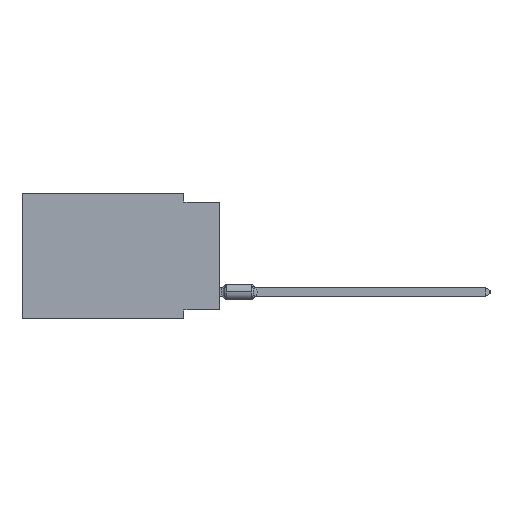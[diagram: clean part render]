
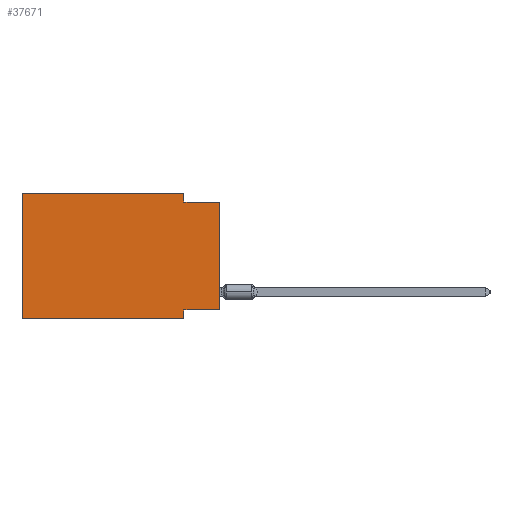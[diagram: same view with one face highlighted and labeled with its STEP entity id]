
A CAD part, left-side view. The second image highlights one B-rep face of the part: STEP entity #37671.
In plain terms, the highlighted planar face has unit normal (-1, 0, 0).
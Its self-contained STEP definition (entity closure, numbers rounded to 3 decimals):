
#9 = EDGE_CURVE ( 'NONE', #63731, #5928, #62238, .T. ) ;
#2051 = CARTESIAN_POINT ( 'NONE',  ( 0., 13.97, -8.89 ) ) ;
#3689 = VECTOR ( 'NONE', #49801, 1000. ) ;
#4534 = EDGE_CURVE ( 'NONE', #6087, #34303, #14583, .T. ) ;
#5928 = VERTEX_POINT ( 'NONE', #48019 ) ;
#6087 = VERTEX_POINT ( 'NONE', #49820 ) ;
#7218 = CARTESIAN_POINT ( 'NONE',  ( 0., 2.54, 0. ) ) ;
#8438 = VERTEX_POINT ( 'NONE', #85431 ) ;
#8828 = CARTESIAN_POINT ( 'NONE',  ( 0., 2.54, -8.89 ) ) ;
#9376 = LINE ( 'NONE', #2051, #74535 ) ;
#9816 = DIRECTION ( 'NONE',  ( 0., -1., 0. ) ) ;
#10262 = ORIENTED_EDGE ( 'NONE', *, *, #72027, .T. ) ;
#13030 = DIRECTION ( 'NONE',  ( 0., 0., -1. ) ) ;
#13647 = VECTOR ( 'NONE', #82854, 1000. ) ;
#14145 = CARTESIAN_POINT ( 'NONE',  ( 0., 0., -0.635 ) ) ;
#14396 = FACE_OUTER_BOUND ( 'NONE', #84794, .T. ) ;
#14546 = VECTOR ( 'NONE', #19195, 1000. ) ;
#14583 = LINE ( 'NONE', #14145, #59259 ) ;
#15708 = DIRECTION ( 'NONE',  ( 0., 0., -1. ) ) ;
#19195 = DIRECTION ( 'NONE',  ( 0., 1., 0. ) ) ;
#19490 = ORIENTED_EDGE ( 'NONE', *, *, #38370, .F. ) ;
#19986 = ORIENTED_EDGE ( 'NONE', *, *, #29115, .F. ) ;
#23646 = CARTESIAN_POINT ( 'NONE',  ( 0., 2.54, -8.89 ) ) ;
#23866 = CARTESIAN_POINT ( 'NONE',  ( 0., 0., -0.635 ) ) ;
#24412 = ORIENTED_EDGE ( 'NONE', *, *, #4534, .F. ) ;
#24677 = VERTEX_POINT ( 'NONE', #23646 ) ;
#25550 = EDGE_CURVE ( 'NONE', #63731, #34303, #51093, .T. ) ;
#27673 = PLANE ( 'NONE',  #41561 ) ;
#29115 = EDGE_CURVE ( 'NONE', #5928, #24677, #35381, .T. ) ;
#34303 = VERTEX_POINT ( 'NONE', #23866 ) ;
#34336 = LINE ( 'NONE', #47635, #13647 ) ;
#35143 = LINE ( 'NONE', #7218, #3689 ) ;
#35381 = LINE ( 'NONE', #8828, #79555 ) ;
#37671 = ADVANCED_FACE ( 'NONE', ( #14396 ), #27673, .F. ) ;
#38094 = CARTESIAN_POINT ( 'NONE',  ( 0., 0., -8.255 ) ) ;
#38370 = EDGE_CURVE ( 'NONE', #76340, #43392, #34336, .T. ) ;
#41561 = AXIS2_PLACEMENT_3D ( 'NONE', #70240, #89934, #13030 ) ;
#43392 = VERTEX_POINT ( 'NONE', #69169 ) ;
#46067 = EDGE_CURVE ( 'NONE', #43392, #8438, #51914, .T. ) ;
#47635 = CARTESIAN_POINT ( 'NONE',  ( 0., 13.97, 0. ) ) ;
#48019 = CARTESIAN_POINT ( 'NONE',  ( 0., 2.54, -8.255 ) ) ;
#49801 = DIRECTION ( 'NONE',  ( 0., 0., -1. ) ) ;
#49820 = CARTESIAN_POINT ( 'NONE',  ( 0., 2.54, -0.635 ) ) ;
#51093 = LINE ( 'NONE', #57066, #71655 ) ;
#51914 = LINE ( 'NONE', #87148, #85048 ) ;
#57066 = CARTESIAN_POINT ( 'NONE',  ( 0., 0., 0. ) ) ;
#58312 = ORIENTED_EDGE ( 'NONE', *, *, #25550, .T. ) ;
#59259 = VECTOR ( 'NONE', #63116, 1000. ) ;
#60447 = CARTESIAN_POINT ( 'NONE',  ( 0., 0., -8.255 ) ) ;
#62238 = LINE ( 'NONE', #60447, #14546 ) ;
#63116 = DIRECTION ( 'NONE',  ( 0., -1., 0. ) ) ;
#63731 = VERTEX_POINT ( 'NONE', #38094 ) ;
#64709 = EDGE_CURVE ( 'NONE', #8438, #6087, #35143, .T. ) ;
#69169 = CARTESIAN_POINT ( 'NONE',  ( 0., 13.97, 0. ) ) ;
#70240 = CARTESIAN_POINT ( 'NONE',  ( 0., 13.97, 0. ) ) ;
#71655 = VECTOR ( 'NONE', #79008, 1000. ) ;
#72027 = EDGE_CURVE ( 'NONE', #76340, #24677, #9376, .T. ) ;
#74535 = VECTOR ( 'NONE', #9816, 1000. ) ;
#76340 = VERTEX_POINT ( 'NONE', #83384 ) ;
#77753 = ORIENTED_EDGE ( 'NONE', *, *, #46067, .F. ) ;
#79008 = DIRECTION ( 'NONE',  ( 0., 0., 1. ) ) ;
#79555 = VECTOR ( 'NONE', #15708, 1000. ) ;
#81544 = ORIENTED_EDGE ( 'NONE', *, *, #64709, .F. ) ;
#82854 = DIRECTION ( 'NONE',  ( 0., 0., 1. ) ) ;
#83384 = CARTESIAN_POINT ( 'NONE',  ( 0., 13.97, -8.89 ) ) ;
#84794 = EDGE_LOOP ( 'NONE', ( #58312, #24412, #81544, #77753, #19490, #10262, #19986, #85507 ) ) ;
#85048 = VECTOR ( 'NONE', #88020, 1000. ) ;
#85431 = CARTESIAN_POINT ( 'NONE',  ( 0., 2.54, 0. ) ) ;
#85507 = ORIENTED_EDGE ( 'NONE', *, *, #9, .F. ) ;
#87148 = CARTESIAN_POINT ( 'NONE',  ( 0., 13.97, 0. ) ) ;
#88020 = DIRECTION ( 'NONE',  ( 0., -1., 0. ) ) ;
#89934 = DIRECTION ( 'NONE',  ( 1., 0., 0. ) ) ;
